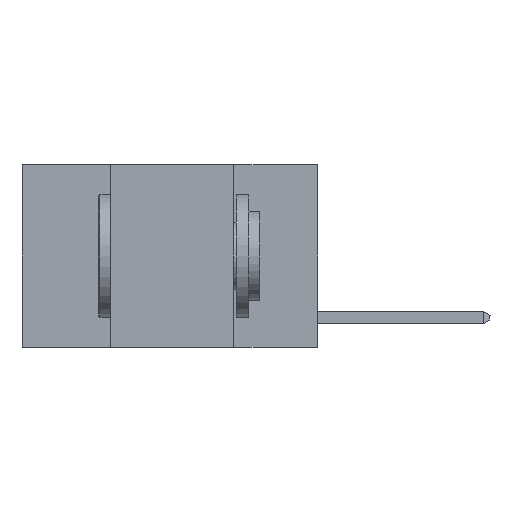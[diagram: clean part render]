
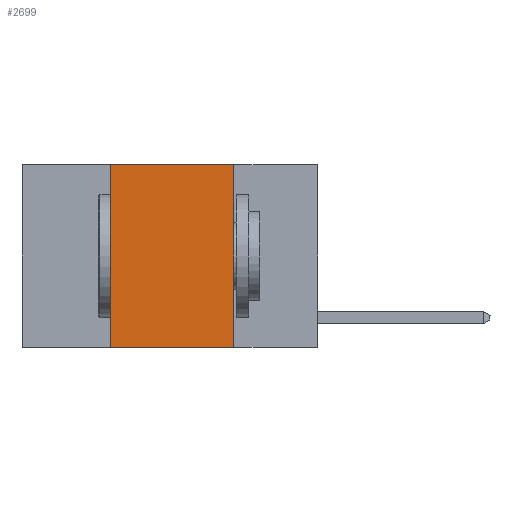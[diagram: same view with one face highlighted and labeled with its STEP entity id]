
A CAD part, left-side view. The second image highlights one B-rep face of the part: STEP entity #2699.
In plain terms, the highlighted planar face has unit normal (-1, 0, 0).
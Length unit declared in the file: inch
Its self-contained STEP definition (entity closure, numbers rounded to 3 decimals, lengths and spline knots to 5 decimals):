
#75 = DIRECTION ( 'NONE',  ( 0., 0., -1. ) ) ;
#254 = VECTOR ( 'NONE', #75, 39.37008 ) ;
#1316 = ORIENTED_EDGE ( 'NONE', *, *, #9558, .F. ) ;
#1423 = FACE_OUTER_BOUND ( 'NONE', #9519, .T. ) ;
#1580 = DIRECTION ( 'NONE',  ( 0., 0., -1. ) ) ;
#1617 = CARTESIAN_POINT ( 'NONE',  ( 0., 0.17, -0.37 ) ) ;
#2168 = AXIS2_PLACEMENT_3D ( 'NONE', #11983, #14931, #1580 ) ;
#2362 = CARTESIAN_POINT ( 'NONE',  ( 0., 0.17, 0. ) ) ;
#2699 = ADVANCED_FACE ( 'NONE', ( #1423 ), #10407, .F. ) ;
#2818 = ORIENTED_EDGE ( 'NONE', *, *, #10064, .F. ) ;
#2833 = ORIENTED_EDGE ( 'NONE', *, *, #13434, .T. ) ;
#3538 = CARTESIAN_POINT ( 'NONE',  ( 0., 0.6, -0.37 ) ) ;
#3854 = CARTESIAN_POINT ( 'NONE',  ( 0., 0.17, 0. ) ) ;
#4035 = VERTEX_POINT ( 'NONE', #10347 ) ;
#5104 = LINE ( 'NONE', #9106, #10504 ) ;
#6527 = CARTESIAN_POINT ( 'NONE',  ( 0., 0.42, -0.37 ) ) ;
#6843 = VECTOR ( 'NONE', #12007, 39.37008 ) ;
#6986 = ORIENTED_EDGE ( 'NONE', *, *, #13303, .F. ) ;
#7420 = DIRECTION ( 'NONE',  ( 0., -1., 0. ) ) ;
#8101 = VERTEX_POINT ( 'NONE', #1617 ) ;
#8190 = LINE ( 'NONE', #13287, #6843 ) ;
#9042 = LINE ( 'NONE', #3854, #254 ) ;
#9106 = CARTESIAN_POINT ( 'NONE',  ( 0., 0.6, 0. ) ) ;
#9519 = EDGE_LOOP ( 'NONE', ( #1316, #2818, #6986, #2833 ) ) ;
#9558 = EDGE_CURVE ( 'NONE', #11636, #8101, #9042, .T. ) ;
#10064 = EDGE_CURVE ( 'NONE', #4035, #11636, #5104, .T. ) ;
#10347 = CARTESIAN_POINT ( 'NONE',  ( 0., 0.42, 0. ) ) ;
#10407 = PLANE ( 'NONE',  #2168 ) ;
#10504 = VECTOR ( 'NONE', #11527, 39.37008 ) ;
#11091 = VECTOR ( 'NONE', #7420, 39.37008 ) ;
#11527 = DIRECTION ( 'NONE',  ( 0., -1., 0. ) ) ;
#11636 = VERTEX_POINT ( 'NONE', #2362 ) ;
#11983 = CARTESIAN_POINT ( 'NONE',  ( 0., 0.6, 0. ) ) ;
#12007 = DIRECTION ( 'NONE',  ( 0., 0., 1. ) ) ;
#13038 = VERTEX_POINT ( 'NONE', #6527 ) ;
#13287 = CARTESIAN_POINT ( 'NONE',  ( 0., 0.42, 0. ) ) ;
#13303 = EDGE_CURVE ( 'NONE', #13038, #4035, #8190, .T. ) ;
#13434 = EDGE_CURVE ( 'NONE', #13038, #8101, #15047, .T. ) ;
#14931 = DIRECTION ( 'NONE',  ( 1., 0., 0. ) ) ;
#15047 = LINE ( 'NONE', #3538, #11091 ) ;
